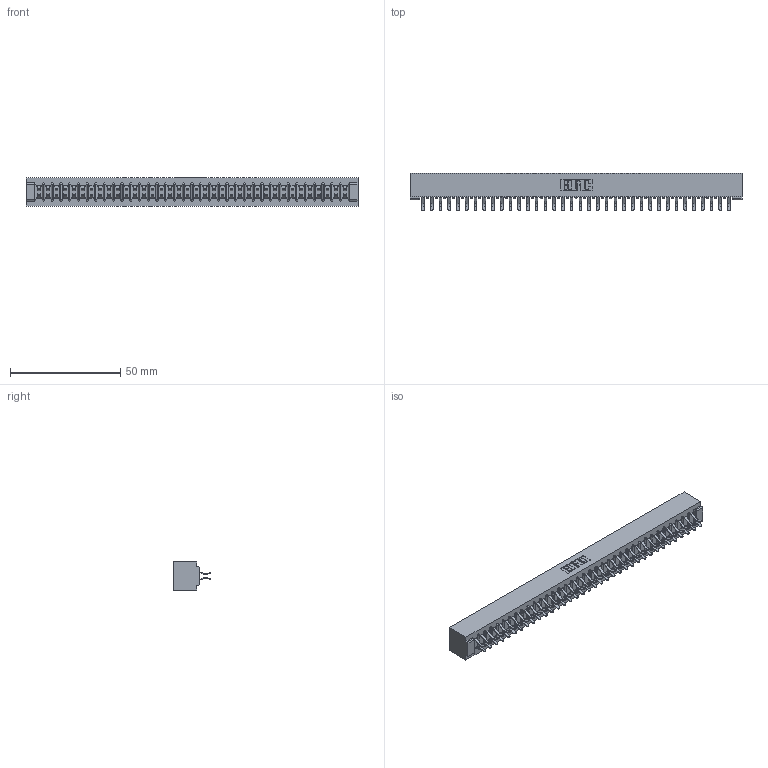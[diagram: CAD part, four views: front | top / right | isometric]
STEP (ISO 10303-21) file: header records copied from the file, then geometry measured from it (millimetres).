
FILE_DESCRIPTION (( 'STEP AP203' ), '1' );
FILE_NAME ('357-072-456-201.STEP', '2020-10-04T19:20:02', ( '' ), ( '' ), 'SwSTEP 2.0', 'SolidWorks 2020', '' );
FILE_SCHEMA (( 'CONFIG_CONTROL_DESIGN' ));
Length unit declared in the file: inch
Products named in the file (3): 357-072-456-201; 307 Part_No Mounting Lugs; 307-290-001_556
Assembly tree (73 placements, depth 2):
  357-072-456-201
    307 Part_No Mounting Lugs
    307-290-001_556  x72
Bounding box: 150.52 x 16.97 x 12.7 mm (x, y, z)
Volume: 16498 mm3; surface area: 20190.5 mm2
Topology: 73 solids, 73 shells, 3747 faces, 10523 edges, 6818 vertices
Faces by surface type: plane 2442, cylinder 1231, sphere 74
Entity records: 32580 total; most frequent: CARTESIAN_POINT 5328, ORIENTED_EDGE 5278, DIRECTION 5221, EDGE_CURVE 2639, LINE 2023, VECTOR 2023, VERTEX_POINT 1706, AXIS2_PLACEMENT_3D 1599
